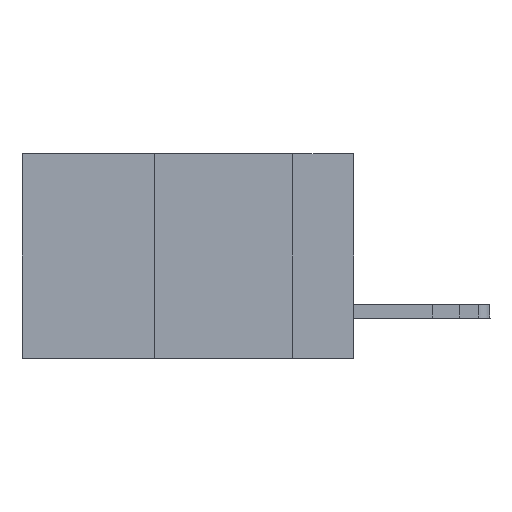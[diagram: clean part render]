
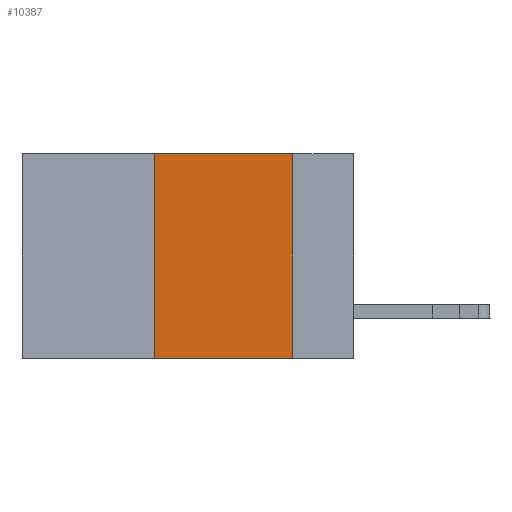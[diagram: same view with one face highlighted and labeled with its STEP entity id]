
A CAD part, left-side view. The second image highlights one B-rep face of the part: STEP entity #10387.
In plain terms, the highlighted planar face has unit normal (-1, 0, 0).
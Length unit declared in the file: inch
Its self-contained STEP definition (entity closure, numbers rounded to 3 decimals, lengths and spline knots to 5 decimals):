
#945 = DIRECTION ( 'NONE',  ( 0., -1., 0. ) ) ;
#1184 = VECTOR ( 'NONE', #22510, 39.37008 ) ;
#2146 = EDGE_CURVE ( 'NONE', #5160, #12067, #35750, .T. ) ;
#4245 = VECTOR ( 'NONE', #15197, 39.37008 ) ;
#5160 = VERTEX_POINT ( 'NONE', #26194 ) ;
#5385 = DIRECTION ( 'NONE',  ( 1., 0., 0. ) ) ;
#5642 = ORIENTED_EDGE ( 'NONE', *, *, #25799, .F. ) ;
#7697 = PLANE ( 'NONE',  #25880 ) ;
#9222 = DIRECTION ( 'NONE',  ( 0., 0., -1. ) ) ;
#10387 = ADVANCED_FACE ( 'NONE', ( #19286 ), #7697, .F. ) ;
#11543 = VECTOR ( 'NONE', #9222, 39.37008 ) ;
#12045 = LINE ( 'NONE', #26540, #11543 ) ;
#12067 = VERTEX_POINT ( 'NONE', #32119 ) ;
#12538 = LINE ( 'NONE', #24155, #4245 ) ;
#13934 = VECTOR ( 'NONE', #945, 39.37008 ) ;
#14167 = CARTESIAN_POINT ( 'NONE',  ( 0., 0.6, 0. ) ) ;
#14310 = LINE ( 'NONE', #23066, #1184 ) ;
#15197 = DIRECTION ( 'NONE',  ( 0., 0., 1. ) ) ;
#17436 = EDGE_CURVE ( 'NONE', #18648, #12067, #12045, .T. ) ;
#17747 = EDGE_CURVE ( 'NONE', #36649, #18648, #14310, .T. ) ;
#18005 = ORIENTED_EDGE ( 'NONE', *, *, #17747, .F. ) ;
#18648 = VERTEX_POINT ( 'NONE', #19353 ) ;
#19286 = FACE_OUTER_BOUND ( 'NONE', #32840, .T. ) ;
#19353 = CARTESIAN_POINT ( 'NONE',  ( 0., 0.11, 0. ) ) ;
#22510 = DIRECTION ( 'NONE',  ( 0., -1., 0. ) ) ;
#23066 = CARTESIAN_POINT ( 'NONE',  ( 0., 0.6, 0. ) ) ;
#24155 = CARTESIAN_POINT ( 'NONE',  ( 0., 0.36, 0. ) ) ;
#25025 = DIRECTION ( 'NONE',  ( 0., 0., -1. ) ) ;
#25799 = EDGE_CURVE ( 'NONE', #5160, #36649, #12538, .T. ) ;
#25880 = AXIS2_PLACEMENT_3D ( 'NONE', #14167, #5385, #25025 ) ;
#26194 = CARTESIAN_POINT ( 'NONE',  ( 0., 0.36, -0.37 ) ) ;
#26287 = ORIENTED_EDGE ( 'NONE', *, *, #2146, .T. ) ;
#26540 = CARTESIAN_POINT ( 'NONE',  ( 0., 0.11, 0. ) ) ;
#27930 = ORIENTED_EDGE ( 'NONE', *, *, #17436, .F. ) ;
#29098 = CARTESIAN_POINT ( 'NONE',  ( 0., 0.36, 0. ) ) ;
#30393 = CARTESIAN_POINT ( 'NONE',  ( 0., 0.6, -0.37 ) ) ;
#32119 = CARTESIAN_POINT ( 'NONE',  ( 0., 0.11, -0.37 ) ) ;
#32840 = EDGE_LOOP ( 'NONE', ( #27930, #18005, #5642, #26287 ) ) ;
#35750 = LINE ( 'NONE', #30393, #13934 ) ;
#36649 = VERTEX_POINT ( 'NONE', #29098 ) ;
